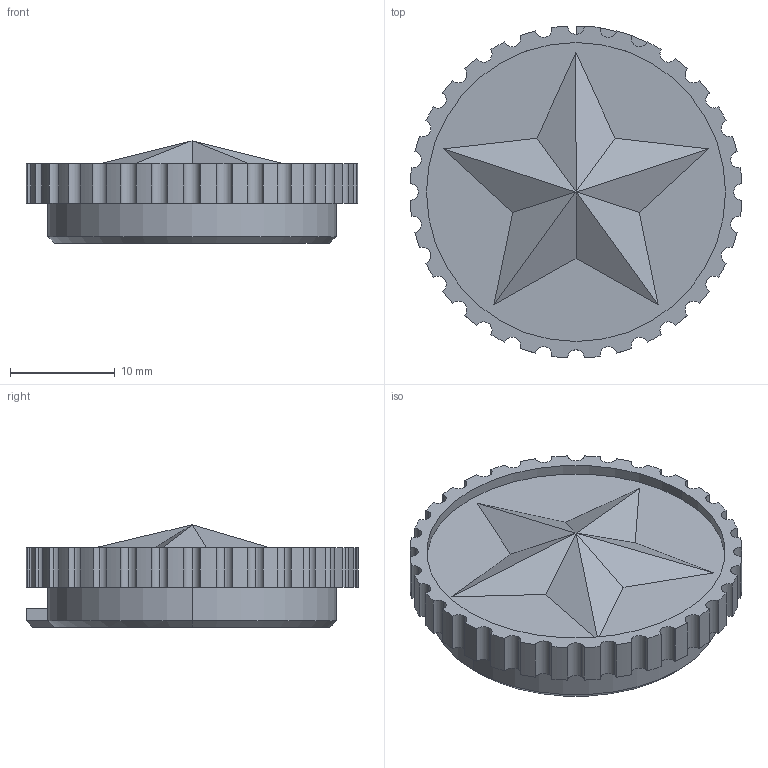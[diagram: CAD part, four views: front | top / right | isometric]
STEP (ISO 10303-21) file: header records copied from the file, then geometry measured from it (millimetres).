
FILE_DESCRIPTION (( 'STEP AP203' ), '1' );
FILE_NAME ('AF-HF-LR-PRT-009-STEP.STEP', '2020-11-04T16:15:53', ( '' ), ( '' ), 'SwSTEP 2.0', 'SolidWorks 2018', '' );
FILE_SCHEMA (( 'CONFIG_CONTROL_DESIGN' ));
Length unit declared in the file: inch
Products named in the file (1): AF-HF-LR-PRT-009-STEP
Bounding box: 31.71 x 31.73 x 9.79 mm (x, y, z)
Volume: 3856.8 mm3; surface area: 2582.3 mm2
Topology: 1 solids, 1 shells, 113 faces, 305 edges, 198 vertices
Faces by surface type: cylinder 86, plane 19, cone 6, sphere 2
Entity records: 3716 total; most frequent: DIRECTION 711, CARTESIAN_POINT 629, ORIENTED_EDGE 610, EDGE_CURVE 305, AXIS2_PLACEMENT_3D 296, VERTEX_POINT 198, CIRCLE 182, LINE 119
